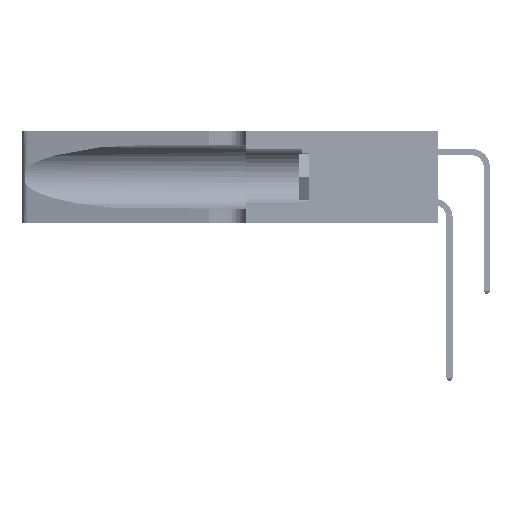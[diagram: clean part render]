
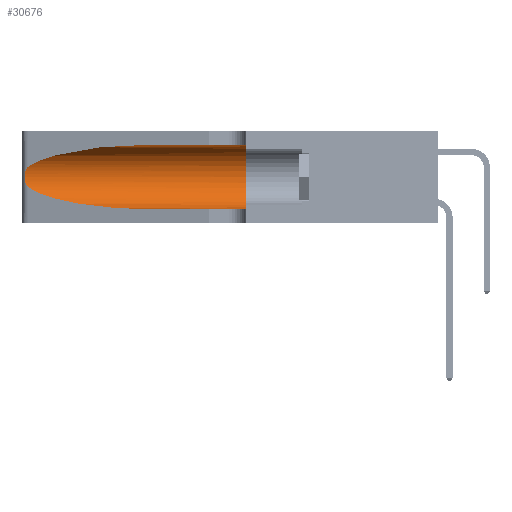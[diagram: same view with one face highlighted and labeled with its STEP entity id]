
A CAD part, left-side view. The second image highlights one B-rep face of the part: STEP entity #30676.
In plain terms, the highlighted cylindrical face has radius 3.308 mm (diameter 6.617 mm), a partial arc.
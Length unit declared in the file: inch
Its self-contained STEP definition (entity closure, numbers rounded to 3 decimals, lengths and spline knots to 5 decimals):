
#515 = DIRECTION ( 'NONE',  ( 0., -1., 0. ) ) ;
#555 = EDGE_CURVE ( 'NONE', #47966, #45811, #51662, .T. ) ;
#902 = EDGE_CURVE ( 'NONE', #47966, #42536, #40691, .T. ) ;
#909 = ORIENTED_EDGE ( 'NONE', *, *, #53077, .T. ) ;
#2382 = ORIENTED_EDGE ( 'NONE', *, *, #902, .F. ) ;
#2943 = CARTESIAN_POINT ( 'NONE',  ( 0.18966, 0.96281, 0.05475 ) ) ;
#3319 = CARTESIAN_POINT ( 'NONE',  ( 0.25487, 1.22718, 0.22369 ) ) ;
#3511 = CARTESIAN_POINT ( 'NONE',  ( 0.25487, 1.22718, 0.14631 ) ) ;
#3514 = CARTESIAN_POINT ( 'NONE',  ( 0.25487, 1.22718, 0.14631 ) ) ;
#4838 = DIRECTION ( 'NONE',  ( 0., -1., 0. ) ) ;
#6181 = ORIENTED_EDGE ( 'NONE', *, *, #52636, .F. ) ;
#6268 = VECTOR ( 'NONE', #21094, 39.37008 ) ;
#6638 = VECTOR ( 'NONE', #515, 39.37008 ) ;
#7665 = CARTESIAN_POINT ( 'NONE',  ( 0.25639, 1.23184, 0.21858 ) ) ;
#8979 = CARTESIAN_POINT ( 'NONE',  ( 0.1305, 0.35, 0.05475 ) ) ;
#8986 = DIRECTION ( 'NONE',  ( 0., 0., -1. ) ) ;
#9042 = DIRECTION ( 'NONE',  ( 0., 1., 0. ) ) ;
#9597 = CARTESIAN_POINT ( 'NONE',  ( 0.1305, 0.35, 0.31525 ) ) ;
#12003 = CARTESIAN_POINT ( 'NONE',  ( 0.25854, 1.2359, 0.20912 ) ) ;
#13767 = EDGE_CURVE ( 'NONE', #32131, #26353, #17721, .T. ) ;
#15292 = AXIS2_PLACEMENT_3D ( 'NONE', #47299, #4838, #8986 ) ;
#16301 = CARTESIAN_POINT ( 'NONE',  ( 0.26075, 1.23896, 0.19203 ) ) ;
#16997 = AXIS2_PLACEMENT_3D ( 'NONE', #34643, #9042, #38881 ) ;
#17721 = LINE ( 'NONE', #33585, #6268 ) ;
#20283 = CYLINDRICAL_SURFACE ( 'NONE', #15292, 0.13025 ) ;
#20610 = CARTESIAN_POINT ( 'NONE',  ( 0.26017, 1.23833, 0.17102 ) ) ;
#20867 = CARTESIAN_POINT ( 'NONE',  ( 0.1305, 0.72297, 0.05475 ) ) ;
#21094 = DIRECTION ( 'NONE',  ( 0., -1., 0. ) ) ;
#21636 = FACE_OUTER_BOUND ( 'NONE', #29095, .T. ) ;
#22477 = CARTESIAN_POINT ( 'NONE',  ( 0.25487, 1.22718, 0.22369 ) ) ;
#23835 = CARTESIAN_POINT ( 'NONE',  ( 0.18966, 0.96281, 0.31525 ) ) ;
#24020 = CARTESIAN_POINT ( 'NONE',  ( 0.25487, 1.22718, 0.22369 ) ) ;
#24308 = CIRCLE ( 'NONE', #16997, 0.13025 ) ;
#24345 = CARTESIAN_POINT ( 'NONE',  ( 0.25487, 1.22718, 0.14631 ) ) ;
#24715 = ORIENTED_EDGE ( 'NONE', *, *, #13767, .T. ) ;
#24903 = CARTESIAN_POINT ( 'NONE',  ( 0.25789, 1.23486, 0.15765 ) ) ;
#26353 = VERTEX_POINT ( 'NONE', #8979 ) ;
#28662 = CARTESIAN_POINT ( 'NONE',  ( 0.2373, 1.15595, 0.08982 ) ) ;
#29095 = EDGE_LOOP ( 'NONE', ( #51140, #909, #54729, #24715, #6181, #2382 ) ) ;
#29212 = CARTESIAN_POINT ( 'NONE',  ( 0.25555, 1.22993, 0.14849 ) ) ;
#30676 = ADVANCED_FACE ( 'NONE', ( #21636 ), #20283, .F. ) ;
#32131 = VERTEX_POINT ( 'NONE', #20867 ) ;
#32833 = VERTEX_POINT ( 'NONE', #3511 ) ;
#32912 = CARTESIAN_POINT ( 'NONE',  ( 0.1305, 0.72297, 0.05475 ) ) ;
#33585 = CARTESIAN_POINT ( 'NONE',  ( 0.1305, 1.61858, 0.05475 ) ) ;
#34643 = CARTESIAN_POINT ( 'NONE',  ( 0.1305, 0.35, 0.185 ) ) ;
#37202 = CARTESIAN_POINT ( 'NONE',  ( 0.25555, 1.22994, 0.2215 ) ) ;
#37359 = EDGE_CURVE ( 'NONE', #32833, #32131, #43542, .T. ) ;
#37569 = CARTESIAN_POINT ( 'NONE',  ( 0.25787, 1.23484, 0.2124 ) ) ;
#38881 = DIRECTION ( 'NONE',  ( 0., 0., 1. ) ) ;
#39498 = B_SPLINE_CURVE_WITH_KNOTS ( 'NONE', 3,
 ( #3319, #37202, #7665, #37569, #12003, #41773, #16301, #46007, #20610, #50252, #24903, #54472, #29212, #3514 ),
 .UNSPECIFIED., .F., .F.,
 ( 4, 2, 2, 2, 2, 2, 4 ),
 ( 0., 0.00027, 0.00053, 0.00107, 0.0016, 0.00187, 0.00214 ),
 .UNSPECIFIED. ) ;
#40691 = LINE ( 'NONE', #47313, #6638 ) ;
#41773 = CARTESIAN_POINT ( 'NONE',  ( 0.26018, 1.23835, 0.19895 ) ) ;
#42536 = VERTEX_POINT ( 'NONE', #9597 ) ;
#43542 =( BOUNDED_CURVE ( )  B_SPLINE_CURVE ( 3, ( #24345, #28662, #2943, #32912 ),
 .UNSPECIFIED., .F., .F. ) 
 B_SPLINE_CURVE_WITH_KNOTS ( ( 4, 4 ),
 ( 3.44316, 4.71239 ),
 .UNSPECIFIED. ) 
 CURVE ( )  GEOMETRIC_REPRESENTATION_ITEM ( )  RATIONAL_B_SPLINE_CURVE ( ( 1., 0.87, 0.87, 1. ) ) 
 REPRESENTATION_ITEM ( '' )  );
#45131 = CARTESIAN_POINT ( 'NONE',  ( 0.2373, 1.15595, 0.28018 ) ) ;
#45811 = VERTEX_POINT ( 'NONE', #22477 ) ;
#46007 = CARTESIAN_POINT ( 'NONE',  ( 0.26075, 1.23896, 0.178 ) ) ;
#47299 = CARTESIAN_POINT ( 'NONE',  ( 0.1305, 1.61858, 0.185 ) ) ;
#47313 = CARTESIAN_POINT ( 'NONE',  ( 0.1305, 1.61858, 0.31525 ) ) ;
#47966 = VERTEX_POINT ( 'NONE', #54222 ) ;
#49354 = CARTESIAN_POINT ( 'NONE',  ( 0.1305, 0.72297, 0.31525 ) ) ;
#50252 = CARTESIAN_POINT ( 'NONE',  ( 0.25856, 1.23593, 0.16098 ) ) ;
#51140 = ORIENTED_EDGE ( 'NONE', *, *, #555, .T. ) ;
#51662 =( BOUNDED_CURVE ( )  B_SPLINE_CURVE ( 3, ( #49354, #23835, #45131, #24020 ),
 .UNSPECIFIED., .F., .F. ) 
 B_SPLINE_CURVE_WITH_KNOTS ( ( 4, 4 ),
 ( 1.5708, 2.84003 ),
 .UNSPECIFIED. ) 
 CURVE ( )  GEOMETRIC_REPRESENTATION_ITEM ( )  RATIONAL_B_SPLINE_CURVE ( ( 1., 0.87, 0.87, 1. ) ) 
 REPRESENTATION_ITEM ( '' )  );
#52636 = EDGE_CURVE ( 'NONE', #42536, #26353, #24308, .T. ) ;
#53077 = EDGE_CURVE ( 'NONE', #45811, #32833, #39498, .T. ) ;
#54222 = CARTESIAN_POINT ( 'NONE',  ( 0.1305, 0.72297, 0.31525 ) ) ;
#54472 = CARTESIAN_POINT ( 'NONE',  ( 0.25639, 1.23186, 0.15144 ) ) ;
#54729 = ORIENTED_EDGE ( 'NONE', *, *, #37359, .T. ) ;
